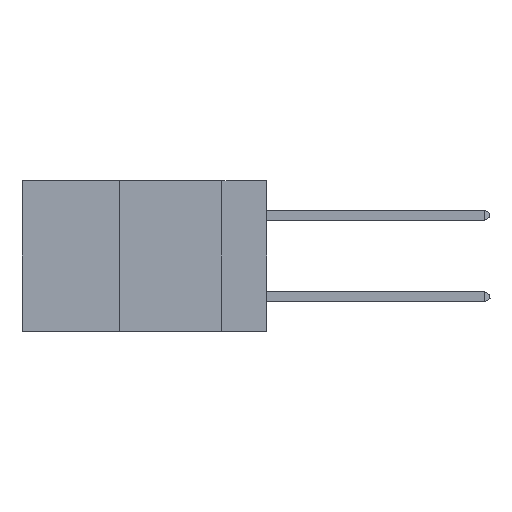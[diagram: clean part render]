
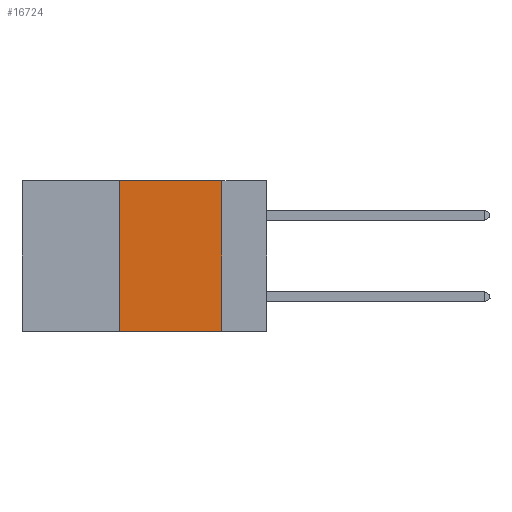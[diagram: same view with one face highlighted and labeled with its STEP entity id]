
A CAD part, left-side view. The second image highlights one B-rep face of the part: STEP entity #16724.
In plain terms, the highlighted planar face has unit normal (-1, 0, 0).
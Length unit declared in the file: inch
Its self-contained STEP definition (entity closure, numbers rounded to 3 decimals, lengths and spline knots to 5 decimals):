
#119 = VERTEX_POINT ( 'NONE', #671 ) ;
#671 = CARTESIAN_POINT ( 'NONE',  ( 0., 0.11, 0. ) ) ;
#720 = EDGE_CURVE ( 'NONE', #119, #21714, #28077, .T. ) ;
#1197 = DIRECTION ( 'NONE',  ( 0., 0., -1. ) ) ;
#1388 = ORIENTED_EDGE ( 'NONE', *, *, #720, .F. ) ;
#3399 = PLANE ( 'NONE',  #10292 ) ;
#4378 = ORIENTED_EDGE ( 'NONE', *, *, #6295, .F. ) ;
#4431 = LINE ( 'NONE', #7082, #19079 ) ;
#6295 = EDGE_CURVE ( 'NONE', #16493, #16167, #4431, .T. ) ;
#7082 = CARTESIAN_POINT ( 'NONE',  ( 0., 0.36, 0. ) ) ;
#9659 = VECTOR ( 'NONE', #17347, 39.37008 ) ;
#10023 = CARTESIAN_POINT ( 'NONE',  ( 0., 0.6, 0. ) ) ;
#10292 = AXIS2_PLACEMENT_3D ( 'NONE', #10023, #16309, #1197 ) ;
#12079 = FACE_OUTER_BOUND ( 'NONE', #17206, .T. ) ;
#13124 = ORIENTED_EDGE ( 'NONE', *, *, #15713, .F. ) ;
#13518 = CARTESIAN_POINT ( 'NONE',  ( 0., 0.6, 0. ) ) ;
#15403 = DIRECTION ( 'NONE',  ( 0., -1., 0. ) ) ;
#15713 = EDGE_CURVE ( 'NONE', #16167, #119, #26566, .T. ) ;
#16167 = VERTEX_POINT ( 'NONE', #17712 ) ;
#16309 = DIRECTION ( 'NONE',  ( 1., 0., 0. ) ) ;
#16493 = VERTEX_POINT ( 'NONE', #17636 ) ;
#16724 = ADVANCED_FACE ( 'NONE', ( #12079 ), #3399, .F. ) ;
#16755 = CARTESIAN_POINT ( 'NONE',  ( 0., 0.11, 0. ) ) ;
#17206 = EDGE_LOOP ( 'NONE', ( #1388, #13124, #4378, #27082 ) ) ;
#17347 = DIRECTION ( 'NONE',  ( 0., -1., 0. ) ) ;
#17636 = CARTESIAN_POINT ( 'NONE',  ( 0., 0.36, -0.37 ) ) ;
#17712 = CARTESIAN_POINT ( 'NONE',  ( 0., 0.36, 0. ) ) ;
#18198 = DIRECTION ( 'NONE',  ( 0., 0., 1. ) ) ;
#19079 = VECTOR ( 'NONE', #18198, 39.37008 ) ;
#19288 = CARTESIAN_POINT ( 'NONE',  ( 0., 0.11, -0.37 ) ) ;
#19541 = LINE ( 'NONE', #24101, #9659 ) ;
#21714 = VERTEX_POINT ( 'NONE', #19288 ) ;
#23494 = DIRECTION ( 'NONE',  ( 0., 0., -1. ) ) ;
#24101 = CARTESIAN_POINT ( 'NONE',  ( 0., 0.6, -0.37 ) ) ;
#25596 = VECTOR ( 'NONE', #23494, 39.37008 ) ;
#26546 = EDGE_CURVE ( 'NONE', #16493, #21714, #19541, .T. ) ;
#26566 = LINE ( 'NONE', #13518, #27125 ) ;
#27082 = ORIENTED_EDGE ( 'NONE', *, *, #26546, .T. ) ;
#27125 = VECTOR ( 'NONE', #15403, 39.37008 ) ;
#28077 = LINE ( 'NONE', #16755, #25596 ) ;
